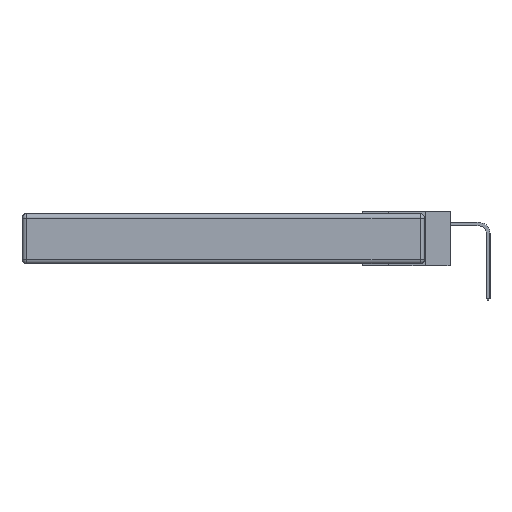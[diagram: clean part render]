
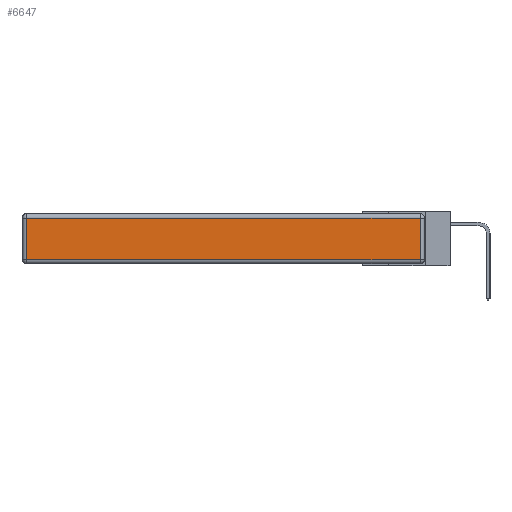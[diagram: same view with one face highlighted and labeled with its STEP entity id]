
A CAD part, left-side view. The second image highlights one B-rep face of the part: STEP entity #6647.
In plain terms, the highlighted planar face has unit normal (-1, 0, 0).
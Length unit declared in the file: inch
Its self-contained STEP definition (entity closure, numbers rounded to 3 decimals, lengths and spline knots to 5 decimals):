
#467 = LINE ( 'NONE', #10043, #17835 ) ;
#783 = DIRECTION ( 'NONE',  ( -1., 0., 0. ) ) ;
#1169 = AXIS2_PLACEMENT_3D ( 'NONE', #14253, #783, #9717 ) ;
#2745 = CARTESIAN_POINT ( 'NONE',  ( 0., 2.72, -0.343 ) ) ;
#2848 = CARTESIAN_POINT ( 'NONE',  ( 0., 0., -0.313 ) ) ;
#3582 = VECTOR ( 'NONE', #23276, 39.37008 ) ;
#5926 = ORIENTED_EDGE ( 'NONE', *, *, #5982, .T. ) ;
#5982 = EDGE_CURVE ( 'NONE', #19136, #15550, #17715, .T. ) ;
#6647 = ADVANCED_FACE ( 'NONE', ( #25753 ), #14353, .T. ) ;
#7913 = ORIENTED_EDGE ( 'NONE', *, *, #16309, .T. ) ;
#9272 = CARTESIAN_POINT ( 'NONE',  ( 0., 0.03, -0.313 ) ) ;
#9717 = DIRECTION ( 'NONE',  ( 0., 0., 1. ) ) ;
#10043 = CARTESIAN_POINT ( 'NONE',  ( 0., 2.75, -0.03 ) ) ;
#12376 = EDGE_CURVE ( 'NONE', #28080, #19136, #13433, .T. ) ;
#13433 = LINE ( 'NONE', #2848, #20122 ) ;
#14253 = CARTESIAN_POINT ( 'NONE',  ( 0., 0., -0.343 ) ) ;
#14353 = PLANE ( 'NONE',  #1169 ) ;
#14868 = VECTOR ( 'NONE', #16385, 39.37008 ) ;
#15460 = EDGE_LOOP ( 'NONE', ( #23021, #5926, #7913, #24300 ) ) ;
#15550 = VERTEX_POINT ( 'NONE', #15759 ) ;
#15759 = CARTESIAN_POINT ( 'NONE',  ( 0., 0.03, -0.03 ) ) ;
#16309 = EDGE_CURVE ( 'NONE', #15550, #26374, #467, .T. ) ;
#16385 = DIRECTION ( 'NONE',  ( 0., 0., 1. ) ) ;
#17715 = LINE ( 'NONE', #20814, #14868 ) ;
#17835 = VECTOR ( 'NONE', #26735, 39.37008 ) ;
#18485 = EDGE_CURVE ( 'NONE', #26374, #28080, #21938, .T. ) ;
#18684 = DIRECTION ( 'NONE',  ( 0., -1., 0. ) ) ;
#19136 = VERTEX_POINT ( 'NONE', #9272 ) ;
#20122 = VECTOR ( 'NONE', #18684, 39.37008 ) ;
#20814 = CARTESIAN_POINT ( 'NONE',  ( 0., 0.03, -0.343 ) ) ;
#21813 = CARTESIAN_POINT ( 'NONE',  ( 0., 2.72, -0.313 ) ) ;
#21938 = LINE ( 'NONE', #2745, #3582 ) ;
#23021 = ORIENTED_EDGE ( 'NONE', *, *, #12376, .T. ) ;
#23276 = DIRECTION ( 'NONE',  ( 0., 0., -1. ) ) ;
#24300 = ORIENTED_EDGE ( 'NONE', *, *, #18485, .T. ) ;
#25753 = FACE_OUTER_BOUND ( 'NONE', #15460, .T. ) ;
#26374 = VERTEX_POINT ( 'NONE', #26375 ) ;
#26375 = CARTESIAN_POINT ( 'NONE',  ( 0., 2.72, -0.03 ) ) ;
#26735 = DIRECTION ( 'NONE',  ( 0., 1., 0. ) ) ;
#28080 = VERTEX_POINT ( 'NONE', #21813 ) ;
